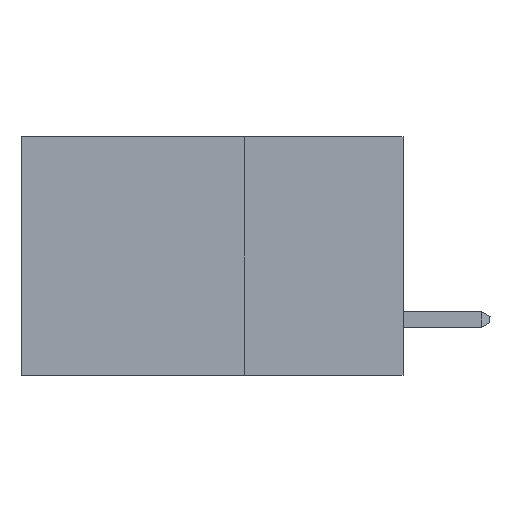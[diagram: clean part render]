
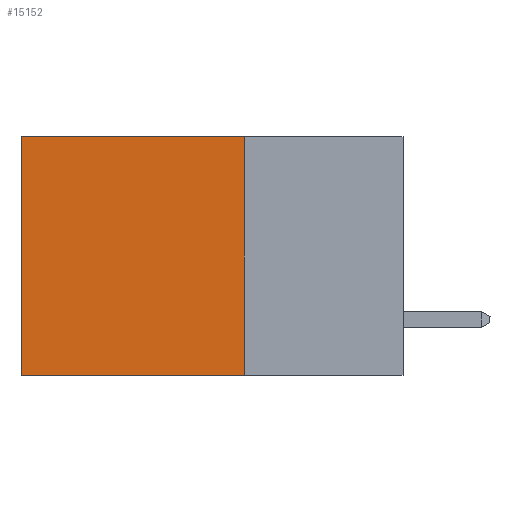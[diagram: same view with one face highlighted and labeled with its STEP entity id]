
A CAD part, left-side view. The second image highlights one B-rep face of the part: STEP entity #15152.
In plain terms, the highlighted planar face has unit normal (-1, 0, 0).
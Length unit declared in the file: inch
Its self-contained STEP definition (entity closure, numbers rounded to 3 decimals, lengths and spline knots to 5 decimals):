
#312 = ORIENTED_EDGE ( 'NONE', *, *, #12635, .F. ) ;
#659 = CARTESIAN_POINT ( 'NONE',  ( 0.2875, 0.25, -0.375 ) ) ;
#738 = CARTESIAN_POINT ( 'NONE',  ( 0.2875, 0.25, 0. ) ) ;
#1791 = CARTESIAN_POINT ( 'NONE',  ( 0.2875, 0.6, -0.375 ) ) ;
#1871 = DIRECTION ( 'NONE',  ( 0., 1., 0. ) ) ;
#3229 = VERTEX_POINT ( 'NONE', #1791 ) ;
#3403 = DIRECTION ( 'NONE',  ( 0., 0., -1. ) ) ;
#3432 = VERTEX_POINT ( 'NONE', #15042 ) ;
#3465 = AXIS2_PLACEMENT_3D ( 'NONE', #659, #9491, #7016 ) ;
#3604 = ORIENTED_EDGE ( 'NONE', *, *, #3813, .T. ) ;
#3791 = EDGE_CURVE ( 'NONE', #5884, #14808, #8202, .T. ) ;
#3813 = EDGE_CURVE ( 'NONE', #3432, #3229, #13093, .T. ) ;
#3838 = VECTOR ( 'NONE', #3403, 39.37008 ) ;
#4630 = DIRECTION ( 'NONE',  ( 0., 0., -1. ) ) ;
#5611 = VECTOR ( 'NONE', #4630, 39.37008 ) ;
#5841 = CARTESIAN_POINT ( 'NONE',  ( 0.2875, 0.6, -0.375 ) ) ;
#5884 = VERTEX_POINT ( 'NONE', #15274 ) ;
#6165 = DIRECTION ( 'NONE',  ( 0., 1., 0. ) ) ;
#6262 = LINE ( 'NONE', #8857, #16270 ) ;
#7016 = DIRECTION ( 'NONE',  ( 0., 0., -1. ) ) ;
#7078 = VECTOR ( 'NONE', #1871, 39.37008 ) ;
#7223 = EDGE_LOOP ( 'NONE', ( #3604, #312, #15226, #9967 ) ) ;
#8202 = LINE ( 'NONE', #9721, #3838 ) ;
#8857 = CARTESIAN_POINT ( 'NONE',  ( 0.2875, 0.25, -0.375 ) ) ;
#9491 = DIRECTION ( 'NONE',  ( 1., 0., 0. ) ) ;
#9567 = EDGE_CURVE ( 'NONE', #5884, #3432, #10412, .T. ) ;
#9721 = CARTESIAN_POINT ( 'NONE',  ( 0.2875, 0.25, -0.375 ) ) ;
#9967 = ORIENTED_EDGE ( 'NONE', *, *, #9567, .T. ) ;
#10412 = LINE ( 'NONE', #738, #7078 ) ;
#11447 = CARTESIAN_POINT ( 'NONE',  ( 0.2875, 0.25, -0.375 ) ) ;
#12635 = EDGE_CURVE ( 'NONE', #14808, #3229, #6262, .T. ) ;
#13093 = LINE ( 'NONE', #5841, #5611 ) ;
#14519 = PLANE ( 'NONE',  #3465 ) ;
#14808 = VERTEX_POINT ( 'NONE', #11447 ) ;
#15042 = CARTESIAN_POINT ( 'NONE',  ( 0.2875, 0.6, 0. ) ) ;
#15152 = ADVANCED_FACE ( 'NONE', ( #15790 ), #14519, .F. ) ;
#15226 = ORIENTED_EDGE ( 'NONE', *, *, #3791, .F. ) ;
#15274 = CARTESIAN_POINT ( 'NONE',  ( 0.2875, 0.25, 0. ) ) ;
#15790 = FACE_OUTER_BOUND ( 'NONE', #7223, .T. ) ;
#16270 = VECTOR ( 'NONE', #6165, 39.37008 ) ;
